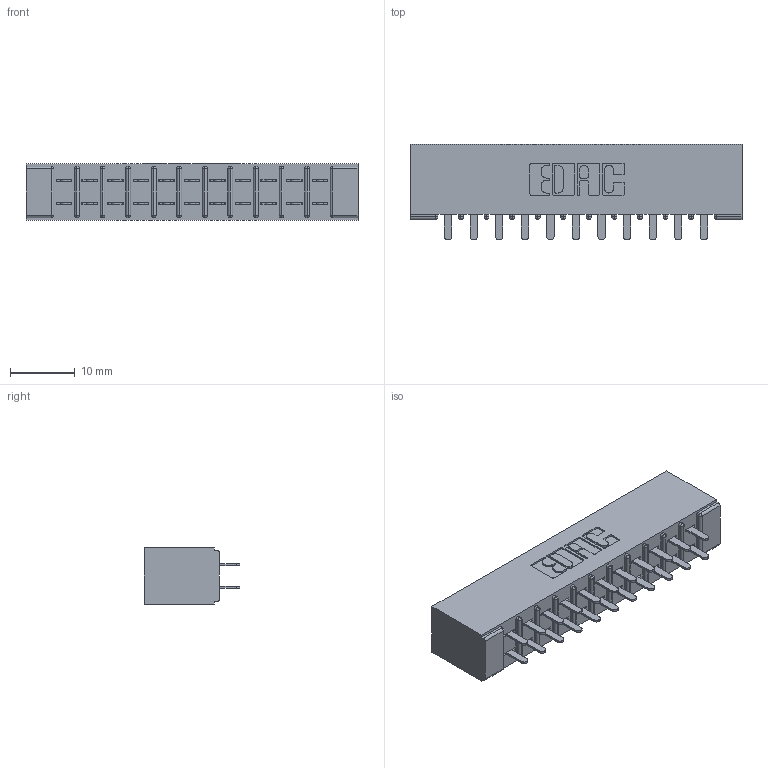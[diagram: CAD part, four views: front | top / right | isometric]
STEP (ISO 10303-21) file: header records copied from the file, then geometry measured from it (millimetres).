
FILE_DESCRIPTION (( 'STEP AP203' ), '1' );
FILE_NAME ('315-022-521-201.STEP', '2019-09-10T14:26:08', ( '' ), ( '' ), 'SwSTEP 2.0', 'SolidWorks 2016', '' );
FILE_SCHEMA (( 'CONFIG_CONTROL_DESIGN' ));
Length unit declared in the file: inch
Products named in the file (3): 305-290-001_521; 305 Part_No Mounting; 315-022-521-201
Assembly tree (23 placements, depth 2):
  315-022-521-201
    305 Part_No Mounting
    305-290-001_521  x22
Bounding box: 51.46 x 14.86 x 8.71 mm (x, y, z)
Volume: 3418.5 mm3; surface area: 6269.3 mm2
Topology: 23 solids, 23 shells, 1120 faces, 3185 edges, 2062 vertices
Faces by surface type: plane 658, cylinder 418, sphere 44
Entity records: 15286 total; most frequent: CARTESIAN_POINT 2527, ORIENTED_EDGE 2502, DIRECTION 2467, EDGE_CURVE 1251, LINE 983, VECTOR 983, VERTEX_POINT 802, AXIS2_PLACEMENT_3D 742
